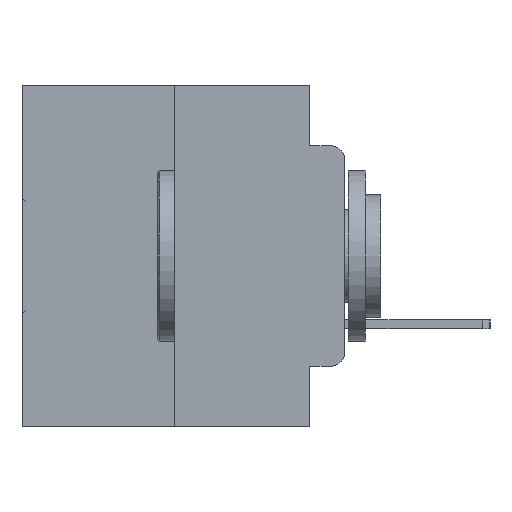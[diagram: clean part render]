
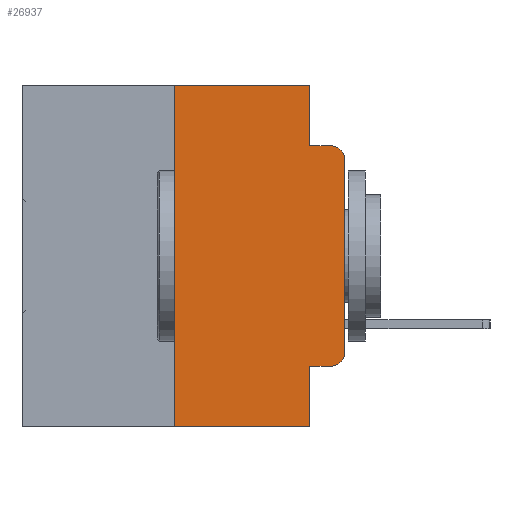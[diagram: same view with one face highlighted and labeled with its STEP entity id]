
A CAD part, left-side view. The second image highlights one B-rep face of the part: STEP entity #26937.
In plain terms, the highlighted planar face has unit normal (-1, 0, 0).
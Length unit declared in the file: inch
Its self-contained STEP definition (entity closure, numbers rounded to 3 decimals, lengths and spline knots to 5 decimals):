
#158 = VECTOR ( 'NONE', #5805, 39.37008 ) ;
#526 = LINE ( 'NONE', #12678, #19578 ) ;
#552 = CARTESIAN_POINT ( 'NONE',  ( 0., 0.02, -0.4115 ) ) ;
#1043 = CIRCLE ( 'NONE', #8743, 0.02 ) ;
#1566 = AXIS2_PLACEMENT_3D ( 'NONE', #24454, #9758, #26885 ) ;
#1679 = VECTOR ( 'NONE', #27867, 39.37008 ) ;
#1859 = ORIENTED_EDGE ( 'NONE', *, *, #28627, .F. ) ;
#2001 = LINE ( 'NONE', #17696, #2784 ) ;
#2263 = EDGE_CURVE ( 'NONE', #23396, #21976, #526, .T. ) ;
#2740 = DIRECTION ( 'NONE',  ( 0., -1., 0. ) ) ;
#2784 = VECTOR ( 'NONE', #2740, 39.37008 ) ;
#3505 = CARTESIAN_POINT ( 'NONE',  ( 0., 0.051, -0.0885 ) ) ;
#3538 = DIRECTION ( 'NONE',  ( -1., 0., 0. ) ) ;
#4340 = CARTESIAN_POINT ( 'NONE',  ( 0., 0., -0.1085 ) ) ;
#4833 = EDGE_LOOP ( 'NONE', ( #10058, #11641, #19748, #7327, #15540, #29881, #19390, #1859, #15161, #28778 ) ) ;
#5216 = CARTESIAN_POINT ( 'NONE',  ( 0., 0.051, 0. ) ) ;
#5805 = DIRECTION ( 'NONE',  ( 0., -1., 0. ) ) ;
#6681 = VERTEX_POINT ( 'NONE', #25376 ) ;
#7185 = VERTEX_POINT ( 'NONE', #27149 ) ;
#7292 = CARTESIAN_POINT ( 'NONE',  ( 0., 0.02, -0.0885 ) ) ;
#7327 = ORIENTED_EDGE ( 'NONE', *, *, #15481, .F. ) ;
#7865 = CARTESIAN_POINT ( 'NONE',  ( 0., 0., 0. ) ) ;
#7985 = EDGE_CURVE ( 'NONE', #17809, #12049, #25413, .T. ) ;
#8511 = LINE ( 'NONE', #7865, #23133 ) ;
#8595 = CARTESIAN_POINT ( 'NONE',  ( 0., 0.25, 0. ) ) ;
#8743 = AXIS2_PLACEMENT_3D ( 'NONE', #10045, #27167, #12591 ) ;
#8957 = AXIS2_PLACEMENT_3D ( 'NONE', #18488, #3538, #20895 ) ;
#9128 = LINE ( 'NONE', #25446, #1679 ) ;
#9648 = PLANE ( 'NONE',  #1566 ) ;
#9758 = DIRECTION ( 'NONE',  ( 1., 0., 0. ) ) ;
#10045 = CARTESIAN_POINT ( 'NONE',  ( 0., 0.02, -0.3915 ) ) ;
#10058 = ORIENTED_EDGE ( 'NONE', *, *, #18829, .T. ) ;
#10450 = CARTESIAN_POINT ( 'NONE',  ( 0., 0.051, -0.5 ) ) ;
#11051 = LINE ( 'NONE', #20453, #24060 ) ;
#11534 = EDGE_CURVE ( 'NONE', #18341, #15231, #2001, .T. ) ;
#11641 = ORIENTED_EDGE ( 'NONE', *, *, #19614, .T. ) ;
#12049 = VERTEX_POINT ( 'NONE', #5216 ) ;
#12591 = DIRECTION ( 'NONE',  ( 0., 0., -1. ) ) ;
#12678 = CARTESIAN_POINT ( 'NONE',  ( 0., 0.051, -0.4115 ) ) ;
#13640 = DIRECTION ( 'NONE',  ( 0., -1., 0. ) ) ;
#14194 = LINE ( 'NONE', #18229, #158 ) ;
#14525 = DIRECTION ( 'NONE',  ( 0., 0., -1. ) ) ;
#15161 = ORIENTED_EDGE ( 'NONE', *, *, #2263, .T. ) ;
#15231 = VERTEX_POINT ( 'NONE', #7292 ) ;
#15481 = EDGE_CURVE ( 'NONE', #12049, #18341, #9128, .T. ) ;
#15540 = ORIENTED_EDGE ( 'NONE', *, *, #7985, .F. ) ;
#15542 = DIRECTION ( 'NONE',  ( 0., 0., 1. ) ) ;
#16098 = EDGE_CURVE ( 'NONE', #6681, #17809, #11051, .T. ) ;
#16214 = LINE ( 'NONE', #21761, #23423 ) ;
#16305 = DIRECTION ( 'NONE',  ( 0., -1., 0. ) ) ;
#17629 = VERTEX_POINT ( 'NONE', #10450 ) ;
#17696 = CARTESIAN_POINT ( 'NONE',  ( 0., 0.051, -0.0885 ) ) ;
#17809 = VERTEX_POINT ( 'NONE', #8595 ) ;
#17885 = DIRECTION ( 'NONE',  ( 0., 0., 1. ) ) ;
#18229 = CARTESIAN_POINT ( 'NONE',  ( 0., 0.473, -0.5 ) ) ;
#18341 = VERTEX_POINT ( 'NONE', #3505 ) ;
#18488 = CARTESIAN_POINT ( 'NONE',  ( 0., 0.02, -0.1085 ) ) ;
#18775 = CARTESIAN_POINT ( 'NONE',  ( 0., 0.473, 0. ) ) ;
#18829 = EDGE_CURVE ( 'NONE', #7185, #21681, #8511, .T. ) ;
#19390 = ORIENTED_EDGE ( 'NONE', *, *, #23403, .T. ) ;
#19578 = VECTOR ( 'NONE', #13640, 39.37008 ) ;
#19614 = EDGE_CURVE ( 'NONE', #21681, #15231, #29955, .T. ) ;
#19748 = ORIENTED_EDGE ( 'NONE', *, *, #11534, .F. ) ;
#20453 = CARTESIAN_POINT ( 'NONE',  ( 0., 0.25, 0. ) ) ;
#20895 = DIRECTION ( 'NONE',  ( 0., 0., -1. ) ) ;
#21681 = VERTEX_POINT ( 'NONE', #4340 ) ;
#21761 = CARTESIAN_POINT ( 'NONE',  ( 0., 0.051, 0. ) ) ;
#21976 = VERTEX_POINT ( 'NONE', #552 ) ;
#22012 = FACE_OUTER_BOUND ( 'NONE', #4833, .T. ) ;
#23133 = VECTOR ( 'NONE', #17885, 39.37008 ) ;
#23396 = VERTEX_POINT ( 'NONE', #27823 ) ;
#23403 = EDGE_CURVE ( 'NONE', #6681, #17629, #14194, .T. ) ;
#23423 = VECTOR ( 'NONE', #14525, 39.37008 ) ;
#24060 = VECTOR ( 'NONE', #15542, 39.37008 ) ;
#24454 = CARTESIAN_POINT ( 'NONE',  ( 0., 0.473, 0. ) ) ;
#25376 = CARTESIAN_POINT ( 'NONE',  ( 0., 0.25, -0.5 ) ) ;
#25413 = LINE ( 'NONE', #18775, #30230 ) ;
#25446 = CARTESIAN_POINT ( 'NONE',  ( 0., 0.051, 0. ) ) ;
#26885 = DIRECTION ( 'NONE',  ( 0., 0., -1. ) ) ;
#26937 = ADVANCED_FACE ( 'NONE', ( #22012 ), #9648, .F. ) ;
#27149 = CARTESIAN_POINT ( 'NONE',  ( 0., 0., -0.3915 ) ) ;
#27167 = DIRECTION ( 'NONE',  ( -1., 0., 0. ) ) ;
#27644 = EDGE_CURVE ( 'NONE', #21976, #7185, #1043, .T. ) ;
#27823 = CARTESIAN_POINT ( 'NONE',  ( 0., 0.051, -0.4115 ) ) ;
#27867 = DIRECTION ( 'NONE',  ( 0., 0., -1. ) ) ;
#28627 = EDGE_CURVE ( 'NONE', #23396, #17629, #16214, .T. ) ;
#28778 = ORIENTED_EDGE ( 'NONE', *, *, #27644, .T. ) ;
#29881 = ORIENTED_EDGE ( 'NONE', *, *, #16098, .F. ) ;
#29955 = CIRCLE ( 'NONE', #8957, 0.02 ) ;
#30230 = VECTOR ( 'NONE', #16305, 39.37008 ) ;
